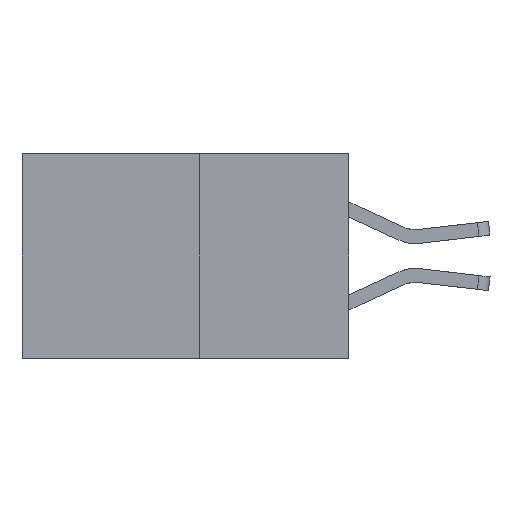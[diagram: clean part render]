
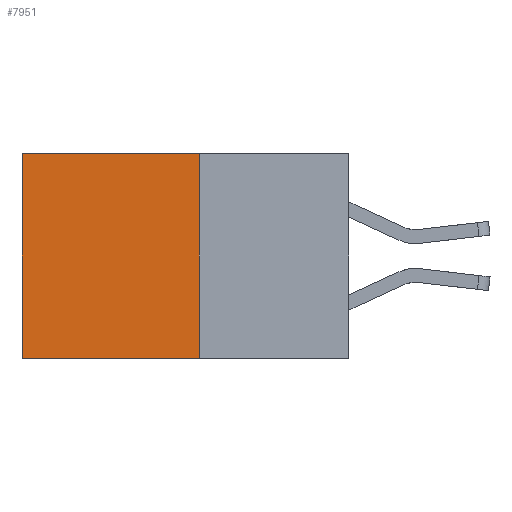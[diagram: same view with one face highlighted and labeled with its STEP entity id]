
A CAD part, left-side view. The second image highlights one B-rep face of the part: STEP entity #7951.
In plain terms, the highlighted planar face has unit normal (-1, 0, 0).
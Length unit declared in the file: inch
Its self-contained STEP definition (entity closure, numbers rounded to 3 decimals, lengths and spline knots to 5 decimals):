
#191 = ORIENTED_EDGE ( 'NONE', *, *, #3384, .T. ) ;
#192 = DIRECTION ( 'NONE',  ( 0., 0., -1. ) ) ;
#699 = DIRECTION ( 'NONE',  ( 0., 1., 0. ) ) ;
#770 = CARTESIAN_POINT ( 'NONE',  ( 0.277, 0.27, -0.37 ) ) ;
#842 = LINE ( 'NONE', #2225, #4324 ) ;
#1214 = VERTEX_POINT ( 'NONE', #1392 ) ;
#1392 = CARTESIAN_POINT ( 'NONE',  ( 0.277, 0.59, -0.37 ) ) ;
#1578 = EDGE_CURVE ( 'NONE', #8396, #6208, #842, .T. ) ;
#1697 = CARTESIAN_POINT ( 'NONE',  ( 0.277, 0.27, 0. ) ) ;
#2225 = CARTESIAN_POINT ( 'NONE',  ( 0.277, 0.27, -0.37 ) ) ;
#2260 = EDGE_CURVE ( 'NONE', #7287, #1214, #4517, .T. ) ;
#2768 = CARTESIAN_POINT ( 'NONE',  ( 0.277, 0.59, 0. ) ) ;
#3070 = EDGE_CURVE ( 'NONE', #6208, #1214, #3524, .T. ) ;
#3373 = DIRECTION ( 'NONE',  ( 1., 0., 0. ) ) ;
#3384 = EDGE_CURVE ( 'NONE', #8396, #7287, #7996, .T. ) ;
#3524 = LINE ( 'NONE', #3938, #7203 ) ;
#3864 = ORIENTED_EDGE ( 'NONE', *, *, #2260, .T. ) ;
#3938 = CARTESIAN_POINT ( 'NONE',  ( 0.277, 0.27, -0.37 ) ) ;
#4120 = CARTESIAN_POINT ( 'NONE',  ( 0.277, 0.59, -0.37 ) ) ;
#4256 = DIRECTION ( 'NONE',  ( 0., 0., -1. ) ) ;
#4324 = VECTOR ( 'NONE', #192, 39.37008 ) ;
#4517 = LINE ( 'NONE', #4120, #6163 ) ;
#5450 = CARTESIAN_POINT ( 'NONE',  ( 0.277, 0.27, -0.37 ) ) ;
#5455 = AXIS2_PLACEMENT_3D ( 'NONE', #5450, #3373, #8104 ) ;
#5615 = FACE_OUTER_BOUND ( 'NONE', #6610, .T. ) ;
#5891 = ORIENTED_EDGE ( 'NONE', *, *, #3070, .F. ) ;
#6123 = PLANE ( 'NONE',  #5455 ) ;
#6163 = VECTOR ( 'NONE', #4256, 39.37008 ) ;
#6208 = VERTEX_POINT ( 'NONE', #770 ) ;
#6460 = VECTOR ( 'NONE', #8395, 39.37008 ) ;
#6610 = EDGE_LOOP ( 'NONE', ( #3864, #5891, #6930, #191 ) ) ;
#6930 = ORIENTED_EDGE ( 'NONE', *, *, #1578, .F. ) ;
#7203 = VECTOR ( 'NONE', #699, 39.37008 ) ;
#7287 = VERTEX_POINT ( 'NONE', #2768 ) ;
#7951 = ADVANCED_FACE ( 'NONE', ( #5615 ), #6123, .F. ) ;
#7996 = LINE ( 'NONE', #8279, #6460 ) ;
#8104 = DIRECTION ( 'NONE',  ( 0., 0., -1. ) ) ;
#8279 = CARTESIAN_POINT ( 'NONE',  ( 0.277, 0.27, 0. ) ) ;
#8395 = DIRECTION ( 'NONE',  ( 0., 1., 0. ) ) ;
#8396 = VERTEX_POINT ( 'NONE', #1697 ) ;
